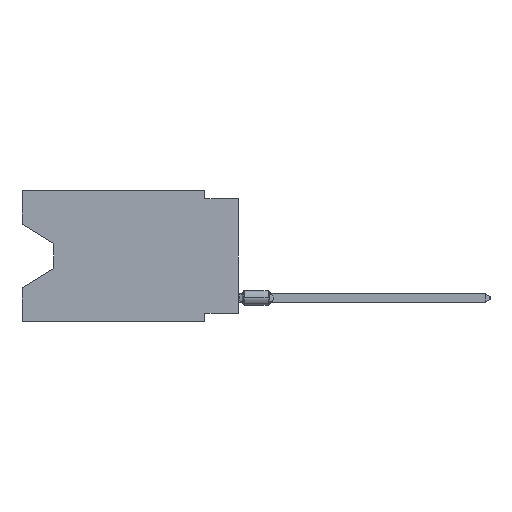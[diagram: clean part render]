
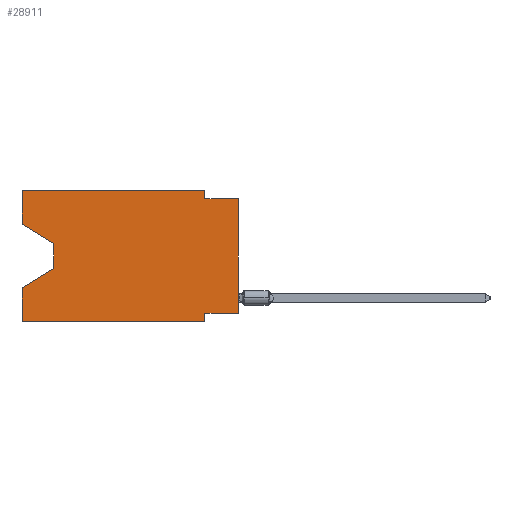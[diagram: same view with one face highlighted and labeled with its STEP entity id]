
A CAD part, left-side view. The second image highlights one B-rep face of the part: STEP entity #28911.
In plain terms, the highlighted planar face has unit normal (-1, 0, 0).
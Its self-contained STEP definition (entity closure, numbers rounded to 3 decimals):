
#11 = EDGE_CURVE ( 'NONE', #38195, #3302, #3607, .T. ) ;
#631 = DIRECTION ( 'NONE',  ( 0., 0., -1. ) ) ;
#654 = EDGE_CURVE ( 'NONE', #16603, #11856, #24596, .T. ) ;
#731 = ORIENTED_EDGE ( 'NONE', *, *, #35711, .T. ) ;
#919 = VECTOR ( 'NONE', #29464, 1000. ) ;
#1276 = CARTESIAN_POINT ( 'NONE',  ( 0., 16.383, -2.546 ) ) ;
#1974 = CARTESIAN_POINT ( 'NONE',  ( 0., 0., 0. ) ) ;
#2188 = CARTESIAN_POINT ( 'NONE',  ( 0., 16.383, 0. ) ) ;
#2283 = VECTOR ( 'NONE', #17591, 1000. ) ;
#2728 = EDGE_CURVE ( 'NONE', #3302, #21091, #28483, .T. ) ;
#2731 = CARTESIAN_POINT ( 'NONE',  ( 0., 2.54, -0.635 ) ) ;
#3302 = VERTEX_POINT ( 'NONE', #27252 ) ;
#3384 = ORIENTED_EDGE ( 'NONE', *, *, #26603, .F. ) ;
#3607 = LINE ( 'NONE', #27395, #23741 ) ;
#3827 = ORIENTED_EDGE ( 'NONE', *, *, #23486, .F. ) ;
#4022 = DIRECTION ( 'NONE',  ( 0., 0.855, -0.519 ) ) ;
#4263 = CARTESIAN_POINT ( 'NONE',  ( 0., 13.97, -4.013 ) ) ;
#5334 = PLANE ( 'NONE',  #9102 ) ;
#5583 = ORIENTED_EDGE ( 'NONE', *, *, #35274, .T. ) ;
#6089 = CARTESIAN_POINT ( 'NONE',  ( 0., 0., -0.635 ) ) ;
#6172 = DIRECTION ( 'NONE',  ( 0., -1., 0. ) ) ;
#8332 = EDGE_CURVE ( 'NONE', #17898, #16603, #33212, .T. ) ;
#8353 = LINE ( 'NONE', #38409, #30978 ) ;
#8490 = CARTESIAN_POINT ( 'NONE',  ( 0., 16.383, 0. ) ) ;
#8704 = FACE_OUTER_BOUND ( 'NONE', #32680, .T. ) ;
#9102 = AXIS2_PLACEMENT_3D ( 'NONE', #2188, #32452, #31854 ) ;
#9755 = LINE ( 'NONE', #25456, #13467 ) ;
#10363 = EDGE_CURVE ( 'NONE', #16026, #11416, #8353, .T. ) ;
#10876 = CARTESIAN_POINT ( 'NONE',  ( 0., 0., -0.635 ) ) ;
#11211 = ORIENTED_EDGE ( 'NONE', *, *, #2728, .F. ) ;
#11416 = VERTEX_POINT ( 'NONE', #20096 ) ;
#11474 = VECTOR ( 'NONE', #20668, 1000. ) ;
#11856 = VERTEX_POINT ( 'NONE', #20826 ) ;
#12191 = CARTESIAN_POINT ( 'NONE',  ( 0., 16.383, 0. ) ) ;
#12517 = ORIENTED_EDGE ( 'NONE', *, *, #28910, .F. ) ;
#13467 = VECTOR ( 'NONE', #4022, 1000. ) ;
#14168 = DIRECTION ( 'NONE',  ( 0., 0., -1. ) ) ;
#14202 = VECTOR ( 'NONE', #20486, 1000. ) ;
#14693 = VERTEX_POINT ( 'NONE', #37555 ) ;
#15181 = LINE ( 'NONE', #27134, #14202 ) ;
#15438 = EDGE_CURVE ( 'NONE', #21091, #16710, #38169, .T. ) ;
#16026 = VERTEX_POINT ( 'NONE', #18314 ) ;
#16603 = VERTEX_POINT ( 'NONE', #4263 ) ;
#16710 = VERTEX_POINT ( 'NONE', #6089 ) ;
#17352 = CARTESIAN_POINT ( 'NONE',  ( 0., 16.383, -2.546 ) ) ;
#17591 = DIRECTION ( 'NONE',  ( 0., -1., 0. ) ) ;
#17898 = VERTEX_POINT ( 'NONE', #1276 ) ;
#18314 = CARTESIAN_POINT ( 'NONE',  ( 0., 16.383, -9.906 ) ) ;
#19144 = ORIENTED_EDGE ( 'NONE', *, *, #11, .F. ) ;
#20096 = CARTESIAN_POINT ( 'NONE',  ( 0., 2.54, -9.906 ) ) ;
#20486 = DIRECTION ( 'NONE',  ( 0., 1., 0. ) ) ;
#20668 = DIRECTION ( 'NONE',  ( 0., 0., 1. ) ) ;
#20826 = CARTESIAN_POINT ( 'NONE',  ( 0., 13.97, -5.893 ) ) ;
#21091 = VERTEX_POINT ( 'NONE', #2731 ) ;
#21511 = ORIENTED_EDGE ( 'NONE', *, *, #10363, .T. ) ;
#21909 = VECTOR ( 'NONE', #631, 1000. ) ;
#21934 = ORIENTED_EDGE ( 'NONE', *, *, #30739, .F. ) ;
#23486 = EDGE_CURVE ( 'NONE', #32447, #11416, #23851, .T. ) ;
#23504 = DIRECTION ( 'NONE',  ( 0., -1., 0. ) ) ;
#23741 = VECTOR ( 'NONE', #6172, 1000. ) ;
#23851 = LINE ( 'NONE', #33045, #37687 ) ;
#24539 = CARTESIAN_POINT ( 'NONE',  ( 0., 2.54, -9.271 ) ) ;
#24596 = LINE ( 'NONE', #27917, #21909 ) ;
#25223 = ORIENTED_EDGE ( 'NONE', *, *, #8332, .T. ) ;
#25456 = CARTESIAN_POINT ( 'NONE',  ( 0., 13.97, -5.893 ) ) ;
#25931 = CARTESIAN_POINT ( 'NONE',  ( 0., 2.54, 0. ) ) ;
#26019 = VERTEX_POINT ( 'NONE', #26360 ) ;
#26158 = LINE ( 'NONE', #1974, #919 ) ;
#26187 = DIRECTION ( 'NONE',  ( 0., 0., 1. ) ) ;
#26360 = CARTESIAN_POINT ( 'NONE',  ( 0., 0., -9.271 ) ) ;
#26603 = EDGE_CURVE ( 'NONE', #17898, #38195, #35541, .T. ) ;
#27134 = CARTESIAN_POINT ( 'NONE',  ( 0., 0., -9.271 ) ) ;
#27252 = CARTESIAN_POINT ( 'NONE',  ( 0., 2.54, 0. ) ) ;
#27395 = CARTESIAN_POINT ( 'NONE',  ( 0., 16.383, 0. ) ) ;
#27917 = CARTESIAN_POINT ( 'NONE',  ( 0., 13.97, -4.013 ) ) ;
#28483 = LINE ( 'NONE', #25931, #38646 ) ;
#28910 = EDGE_CURVE ( 'NONE', #16026, #14693, #32238, .T. ) ;
#28911 = ADVANCED_FACE ( 'NONE', ( #8704 ), #5334, .F. ) ;
#29464 = DIRECTION ( 'NONE',  ( 0., 0., 1. ) ) ;
#29858 = DIRECTION ( 'NONE',  ( 0., -0.855, -0.519 ) ) ;
#30407 = VECTOR ( 'NONE', #26187, 1000. ) ;
#30497 = VECTOR ( 'NONE', #29858, 1000. ) ;
#30739 = EDGE_CURVE ( 'NONE', #26019, #32447, #15181, .T. ) ;
#30978 = VECTOR ( 'NONE', #23504, 1000. ) ;
#31854 = DIRECTION ( 'NONE',  ( 0., 0., -1. ) ) ;
#32238 = LINE ( 'NONE', #8490, #30407 ) ;
#32447 = VERTEX_POINT ( 'NONE', #24539 ) ;
#32452 = DIRECTION ( 'NONE',  ( 1., 0., 0. ) ) ;
#32663 = DIRECTION ( 'NONE',  ( 0., 0., -1. ) ) ;
#32680 = EDGE_LOOP ( 'NONE', ( #25223, #32702, #5583, #12517, #21511, #3827, #21934, #731, #36471, #11211, #19144, #3384 ) ) ;
#32702 = ORIENTED_EDGE ( 'NONE', *, *, #654, .T. ) ;
#33045 = CARTESIAN_POINT ( 'NONE',  ( 0., 2.54, -9.906 ) ) ;
#33212 = LINE ( 'NONE', #17352, #30497 ) ;
#35274 = EDGE_CURVE ( 'NONE', #11856, #14693, #9755, .T. ) ;
#35541 = LINE ( 'NONE', #12191, #11474 ) ;
#35711 = EDGE_CURVE ( 'NONE', #26019, #16710, #26158, .T. ) ;
#36471 = ORIENTED_EDGE ( 'NONE', *, *, #15438, .F. ) ;
#37555 = CARTESIAN_POINT ( 'NONE',  ( 0., 16.383, -7.36 ) ) ;
#37687 = VECTOR ( 'NONE', #32663, 1000. ) ;
#37891 = CARTESIAN_POINT ( 'NONE',  ( 0., 16.383, 0. ) ) ;
#38169 = LINE ( 'NONE', #10876, #2283 ) ;
#38195 = VERTEX_POINT ( 'NONE', #37891 ) ;
#38409 = CARTESIAN_POINT ( 'NONE',  ( 0., 16.383, -9.906 ) ) ;
#38646 = VECTOR ( 'NONE', #14168, 1000. ) ;
